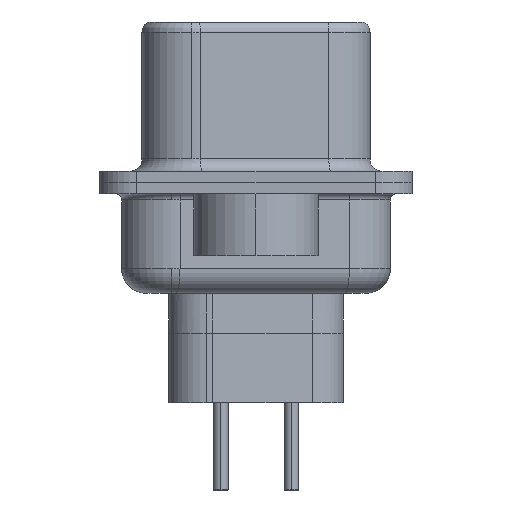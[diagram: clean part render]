
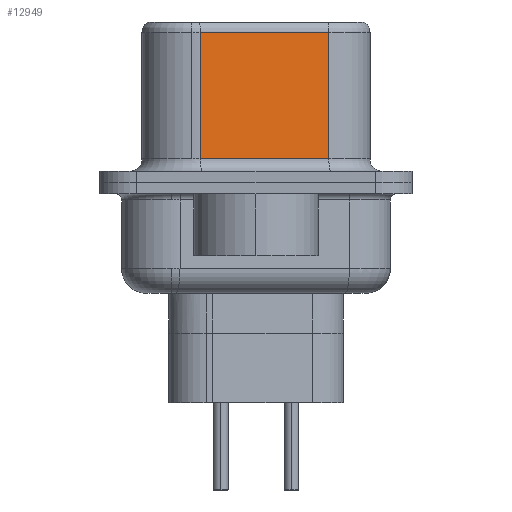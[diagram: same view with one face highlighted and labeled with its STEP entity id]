
A CAD part, left-side view. The second image highlights one B-rep face of the part: STEP entity #12949.
In plain terms, the highlighted planar face has unit normal (-0.985, -0.174, 0).
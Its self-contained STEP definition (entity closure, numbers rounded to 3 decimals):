
#188 = DIRECTION ( 'NONE',  ( -0.174, 0.985, 0. ) ) ;
#817 = EDGE_CURVE ( 'NONE', #22794, #15373, #22358, .T. ) ;
#864 = ORIENTED_EDGE ( 'NONE', *, *, #817, .F. ) ;
#1335 = EDGE_CURVE ( 'NONE', #22794, #24617, #17169, .T. ) ;
#1391 = DIRECTION ( 'NONE',  ( 0., 0., -1. ) ) ;
#3462 = CARTESIAN_POINT ( 'NONE',  ( 4.58, -2.927, 6.52 ) ) ;
#3477 = EDGE_CURVE ( 'NONE', #9912, #15373, #20696, .T. ) ;
#3612 = LINE ( 'NONE', #6068, #19944 ) ;
#3737 = DIRECTION ( 'NONE',  ( 0.174, -0.985, 0. ) ) ;
#3994 = DIRECTION ( 'NONE',  ( 0.985, 0.174, 0. ) ) ;
#4395 = FACE_OUTER_BOUND ( 'NONE', #19750, .T. ) ;
#4476 = CARTESIAN_POINT ( 'NONE',  ( 4.58, -2.927, 6.02 ) ) ;
#4496 = ORIENTED_EDGE ( 'NONE', *, *, #1335, .T. ) ;
#6068 = CARTESIAN_POINT ( 'NONE',  ( 3.67, 2.233, 6.52 ) ) ;
#6928 = AXIS2_PLACEMENT_3D ( 'NONE', #18507, #3994, #23151 ) ;
#8188 = VECTOR ( 'NONE', #188, 1000. ) ;
#8524 = PLANE ( 'NONE',  #6928 ) ;
#9912 = VERTEX_POINT ( 'NONE', #26296 ) ;
#11196 = VECTOR ( 'NONE', #1391, 1000. ) ;
#12949 = ADVANCED_FACE ( 'NONE', ( #4395 ), #8524, .F. ) ;
#15293 = CARTESIAN_POINT ( 'NONE',  ( 3.67, 2.233, 6.02 ) ) ;
#15373 = VERTEX_POINT ( 'NONE', #22627 ) ;
#16574 = DIRECTION ( 'NONE',  ( 0., 0., -1. ) ) ;
#16956 = ORIENTED_EDGE ( 'NONE', *, *, #3477, .T. ) ;
#17169 = LINE ( 'NONE', #4476, #8188 ) ;
#18507 = CARTESIAN_POINT ( 'NONE',  ( 4.58, -2.927, 6.52 ) ) ;
#19750 = EDGE_LOOP ( 'NONE', ( #864, #4496, #26312, #16956 ) ) ;
#19944 = VECTOR ( 'NONE', #16574, 1000. ) ;
#20446 = CARTESIAN_POINT ( 'NONE',  ( 4.58, -2.927, 0.95 ) ) ;
#20696 = LINE ( 'NONE', #20446, #21584 ) ;
#21584 = VECTOR ( 'NONE', #3737, 1000. ) ;
#22358 = LINE ( 'NONE', #3462, #11196 ) ;
#22627 = CARTESIAN_POINT ( 'NONE',  ( 4.58, -2.927, 0.95 ) ) ;
#22794 = VERTEX_POINT ( 'NONE', #26252 ) ;
#23151 = DIRECTION ( 'NONE',  ( -0.174, 0.985, 0. ) ) ;
#24317 = EDGE_CURVE ( 'NONE', #24617, #9912, #3612, .T. ) ;
#24617 = VERTEX_POINT ( 'NONE', #15293 ) ;
#26252 = CARTESIAN_POINT ( 'NONE',  ( 4.58, -2.927, 6.02 ) ) ;
#26296 = CARTESIAN_POINT ( 'NONE',  ( 3.67, 2.233, 0.95 ) ) ;
#26312 = ORIENTED_EDGE ( 'NONE', *, *, #24317, .T. ) ;
